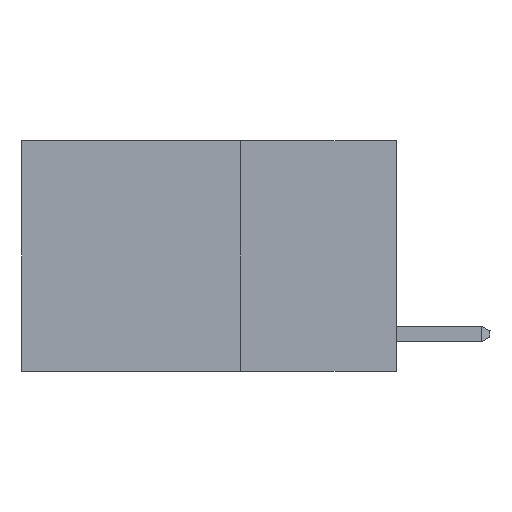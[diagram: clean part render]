
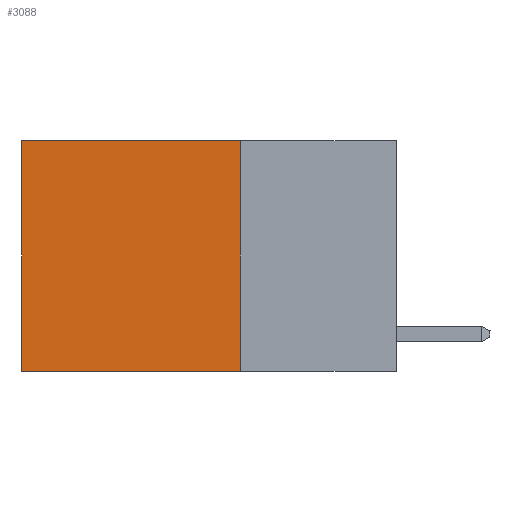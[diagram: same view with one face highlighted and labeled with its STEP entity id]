
A CAD part, left-side view. The second image highlights one B-rep face of the part: STEP entity #3088.
In plain terms, the highlighted planar face has unit normal (-1, 0, 0).
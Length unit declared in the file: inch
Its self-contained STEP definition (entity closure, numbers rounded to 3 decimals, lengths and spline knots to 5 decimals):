
#175 = DIRECTION ( 'NONE',  ( 0., 1., 0. ) ) ;
#293 = VERTEX_POINT ( 'NONE', #3623 ) ;
#822 = VECTOR ( 'NONE', #13568, 39.37008 ) ;
#1173 = EDGE_CURVE ( 'NONE', #12415, #11547, #14168, .T. ) ;
#1447 = LINE ( 'NONE', #7129, #14865 ) ;
#2218 = CARTESIAN_POINT ( 'NONE',  ( 0.2625, 0.6, 0. ) ) ;
#2379 = EDGE_CURVE ( 'NONE', #293, #11547, #1447, .T. ) ;
#2870 = CARTESIAN_POINT ( 'NONE',  ( 0.2625, 0.25, 0. ) ) ;
#3088 = ADVANCED_FACE ( 'NONE', ( #4944 ), #7628, .F. ) ;
#3623 = CARTESIAN_POINT ( 'NONE',  ( 0.2625, 0.25, -0.37 ) ) ;
#4292 = DIRECTION ( 'NONE',  ( 0., 0., -1. ) ) ;
#4444 = VERTEX_POINT ( 'NONE', #2870 ) ;
#4944 = FACE_OUTER_BOUND ( 'NONE', #11544, .T. ) ;
#5378 = VECTOR ( 'NONE', #4292, 39.37008 ) ;
#5634 = LINE ( 'NONE', #8782, #822 ) ;
#6278 = CARTESIAN_POINT ( 'NONE',  ( 0.2625, 0.25, 0. ) ) ;
#6443 = DIRECTION ( 'NONE',  ( 0., 0., -1. ) ) ;
#7129 = CARTESIAN_POINT ( 'NONE',  ( 0.2625, 0.25, -0.37 ) ) ;
#7628 = PLANE ( 'NONE',  #11258 ) ;
#8479 = VECTOR ( 'NONE', #6443, 39.37008 ) ;
#8622 = EDGE_CURVE ( 'NONE', #4444, #293, #14870, .T. ) ;
#8782 = CARTESIAN_POINT ( 'NONE',  ( 0.2625, 0.25, 0. ) ) ;
#9360 = CARTESIAN_POINT ( 'NONE',  ( 0.2625, 0.25, 0. ) ) ;
#9841 = ORIENTED_EDGE ( 'NONE', *, *, #14997, .T. ) ;
#9896 = DIRECTION ( 'NONE',  ( 1., 0., 0. ) ) ;
#10528 = ORIENTED_EDGE ( 'NONE', *, *, #1173, .T. ) ;
#10682 = CARTESIAN_POINT ( 'NONE',  ( 0.2625, 0.6, 0. ) ) ;
#11258 = AXIS2_PLACEMENT_3D ( 'NONE', #6278, #9896, #12294 ) ;
#11544 = EDGE_LOOP ( 'NONE', ( #10528, #12229, #13873, #9841 ) ) ;
#11547 = VERTEX_POINT ( 'NONE', #14106 ) ;
#12229 = ORIENTED_EDGE ( 'NONE', *, *, #2379, .F. ) ;
#12294 = DIRECTION ( 'NONE',  ( 0., 0., -1. ) ) ;
#12415 = VERTEX_POINT ( 'NONE', #10682 ) ;
#13568 = DIRECTION ( 'NONE',  ( 0., 1., 0. ) ) ;
#13873 = ORIENTED_EDGE ( 'NONE', *, *, #8622, .F. ) ;
#14106 = CARTESIAN_POINT ( 'NONE',  ( 0.2625, 0.6, -0.37 ) ) ;
#14168 = LINE ( 'NONE', #2218, #5378 ) ;
#14865 = VECTOR ( 'NONE', #175, 39.37008 ) ;
#14870 = LINE ( 'NONE', #9360, #8479 ) ;
#14997 = EDGE_CURVE ( 'NONE', #4444, #12415, #5634, .T. ) ;
